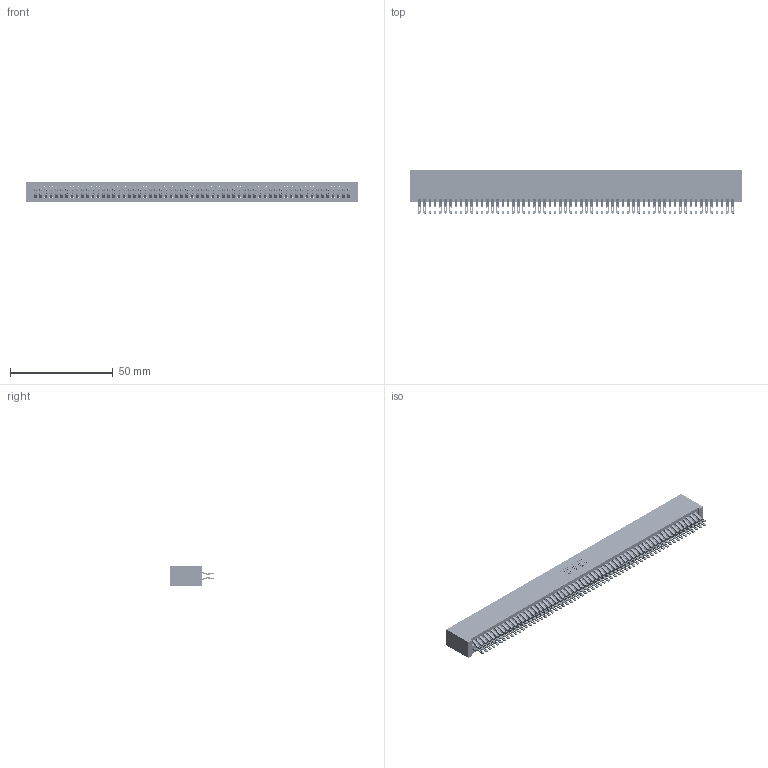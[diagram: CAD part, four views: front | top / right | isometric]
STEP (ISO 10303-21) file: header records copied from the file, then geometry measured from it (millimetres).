
FILE_DESCRIPTION (( 'STEP AP203' ), '1' );
FILE_NAME ('845-122-555-201.STEP', '2018-11-21T12:44:49', ( '' ), ( '' ), 'SwSTEP 2.0', 'SolidWorks 2016', '' );
FILE_SCHEMA (( 'CONFIG_CONTROL_DESIGN' ));
Length unit declared in the file: inch
Products named in the file (3): 845 Part_No Mounting Lugs; 345-292-001_555 Tail; 845-122-555-201
Assembly tree (123 placements, depth 2):
  845-122-555-201
    845 Part_No Mounting Lugs
    345-292-001_555 Tail  x122
Bounding box: 161.54 x 21.13 x 9.4 mm (x, y, z)
Volume: 16838.7 mm3; surface area: 26792.5 mm2
Topology: 123 solids, 123 shells, 6950 faces, 21911 edges, 14606 vertices
Faces by surface type: plane 3858, cylinder 3092
Entity records: 45353 total; most frequent: CARTESIAN_POINT 7618, ORIENTED_EDGE 7522, DIRECTION 6657, EDGE_CURVE 3761, VECTOR 3373, LINE 3373, VERTEX_POINT 2506, AXIS2_PLACEMENT_3D 1642
